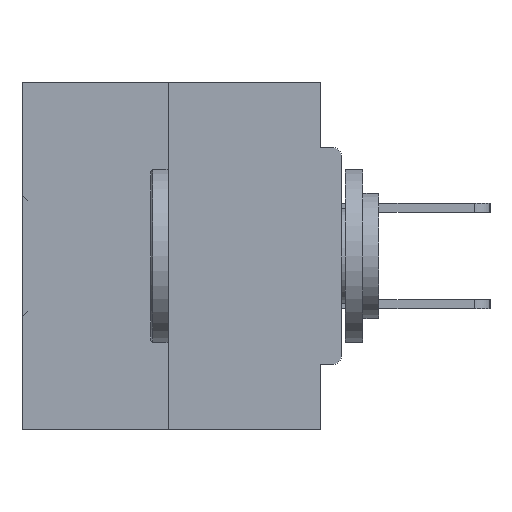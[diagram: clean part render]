
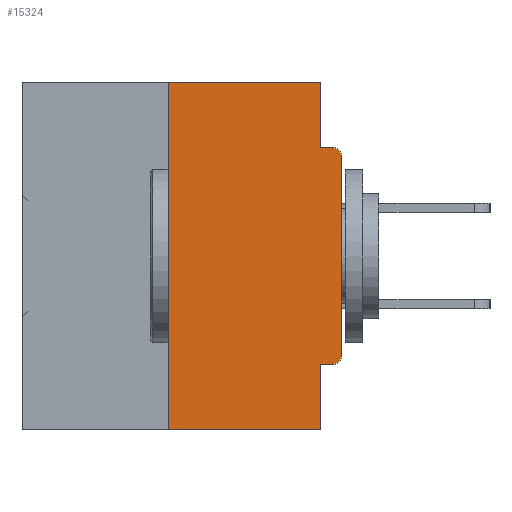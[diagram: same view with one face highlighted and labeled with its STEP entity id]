
A CAD part, left-side view. The second image highlights one B-rep face of the part: STEP entity #15324.
In plain terms, the highlighted planar face has unit normal (-1, 0, 0).
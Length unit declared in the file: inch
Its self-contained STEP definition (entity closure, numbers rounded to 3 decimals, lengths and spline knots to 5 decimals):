
#366 = LINE ( 'NONE', #34120, #34697 ) ;
#752 = AXIS2_PLACEMENT_3D ( 'NONE', #9094, #35102, #16743 ) ;
#790 = DIRECTION ( 'NONE',  ( 0., 1., 0. ) ) ;
#894 = DIRECTION ( 'NONE',  ( 0., -1., 0. ) ) ;
#1002 = ORIENTED_EDGE ( 'NONE', *, *, #1073, .F. ) ;
#1073 = EDGE_CURVE ( 'NONE', #8183, #37751, #38777, .T. ) ;
#2745 = EDGE_CURVE ( 'NONE', #17777, #28330, #366, .T. ) ;
#3215 = AXIS2_PLACEMENT_3D ( 'NONE', #20909, #6775, #28810 ) ;
#4293 = EDGE_CURVE ( 'NONE', #5166, #22107, #28750, .T. ) ;
#4902 = CARTESIAN_POINT ( 'NONE',  ( 0., 0.46, -0.5 ) ) ;
#5001 = DIRECTION ( 'NONE',  ( 0., 0., 1. ) ) ;
#5049 = AXIS2_PLACEMENT_3D ( 'NONE', #6238, #16967, #46202 ) ;
#5166 = VERTEX_POINT ( 'NONE', #45903 ) ;
#6108 = VECTOR ( 'NONE', #5001, 39.37008 ) ;
#6238 = CARTESIAN_POINT ( 'NONE',  ( 0., 0.46, 0. ) ) ;
#6361 = ORIENTED_EDGE ( 'NONE', *, *, #19238, .F. ) ;
#6560 = VERTEX_POINT ( 'NONE', #32976 ) ;
#6732 = CARTESIAN_POINT ( 'NONE',  ( 0., 0.031, -0.0935 ) ) ;
#6775 = DIRECTION ( 'NONE',  ( -1., 0., 0. ) ) ;
#7239 = EDGE_CURVE ( 'NONE', #24102, #6560, #45724, .T. ) ;
#7596 = EDGE_CURVE ( 'NONE', #8183, #22107, #18834, .T. ) ;
#7931 = VECTOR ( 'NONE', #894, 39.37008 ) ;
#8078 = LINE ( 'NONE', #15878, #11506 ) ;
#8183 = VERTEX_POINT ( 'NONE', #12443 ) ;
#8232 = CARTESIAN_POINT ( 'NONE',  ( 0., 0.031, 0. ) ) ;
#9094 = CARTESIAN_POINT ( 'NONE',  ( 0., 0.015, -0.3915 ) ) ;
#9449 = ORIENTED_EDGE ( 'NONE', *, *, #27895, .T. ) ;
#9565 = CARTESIAN_POINT ( 'NONE',  ( 0., 0.031, -0.5 ) ) ;
#11238 = ORIENTED_EDGE ( 'NONE', *, *, #7596, .T. ) ;
#11506 = VECTOR ( 'NONE', #44979, 39.37008 ) ;
#12329 = CARTESIAN_POINT ( 'NONE',  ( 0., 0.25, 0. ) ) ;
#12443 = CARTESIAN_POINT ( 'NONE',  ( 0., 0.25, -0.5 ) ) ;
#13688 = DIRECTION ( 'NONE',  ( 0., 0., -1. ) ) ;
#14679 = VERTEX_POINT ( 'NONE', #15962 ) ;
#15324 = ADVANCED_FACE ( 'NONE', ( #37534 ), #31179, .F. ) ;
#15878 = CARTESIAN_POINT ( 'NONE',  ( 0., 0.031, 0. ) ) ;
#15962 = CARTESIAN_POINT ( 'NONE',  ( 0., 0.015, -0.4065 ) ) ;
#16018 = CARTESIAN_POINT ( 'NONE',  ( 0., 0.46, 0. ) ) ;
#16743 = DIRECTION ( 'NONE',  ( 0., 0., -1. ) ) ;
#16967 = DIRECTION ( 'NONE',  ( 1., 0., 0. ) ) ;
#17101 = CARTESIAN_POINT ( 'NONE',  ( 0., 0., 0. ) ) ;
#17777 = VERTEX_POINT ( 'NONE', #6732 ) ;
#18155 = ORIENTED_EDGE ( 'NONE', *, *, #26161, .F. ) ;
#18808 = EDGE_LOOP ( 'NONE', ( #18155, #1002, #11238, #30719, #33522, #9449, #39337, #42216, #21099, #6361 ) ) ;
#18834 = LINE ( 'NONE', #4902, #7931 ) ;
#19238 = EDGE_CURVE ( 'NONE', #31193, #17777, #8078, .T. ) ;
#19810 = DIRECTION ( 'NONE',  ( 0., -1., 0. ) ) ;
#20909 = CARTESIAN_POINT ( 'NONE',  ( 0., 0.015, -0.1085 ) ) ;
#21099 = ORIENTED_EDGE ( 'NONE', *, *, #2745, .F. ) ;
#21401 = CARTESIAN_POINT ( 'NONE',  ( 0., 0., -0.3915 ) ) ;
#22107 = VERTEX_POINT ( 'NONE', #40289 ) ;
#22546 = VECTOR ( 'NONE', #13688, 39.37008 ) ;
#22756 = CARTESIAN_POINT ( 'NONE',  ( 0., 0., -0.4065 ) ) ;
#23541 = LINE ( 'NONE', #16018, #34956 ) ;
#24102 = VERTEX_POINT ( 'NONE', #21401 ) ;
#24455 = CARTESIAN_POINT ( 'NONE',  ( 0., 0.25, 0. ) ) ;
#26161 = EDGE_CURVE ( 'NONE', #37751, #31193, #23541, .T. ) ;
#27895 = EDGE_CURVE ( 'NONE', #14679, #24102, #35081, .T. ) ;
#28124 = LINE ( 'NONE', #22756, #32124 ) ;
#28330 = VERTEX_POINT ( 'NONE', #41328 ) ;
#28750 = LINE ( 'NONE', #9565, #22546 ) ;
#28810 = DIRECTION ( 'NONE',  ( 0., 0., -1. ) ) ;
#30719 = ORIENTED_EDGE ( 'NONE', *, *, #4293, .F. ) ;
#31179 = PLANE ( 'NONE',  #5049 ) ;
#31193 = VERTEX_POINT ( 'NONE', #8232 ) ;
#31375 = VECTOR ( 'NONE', #46331, 39.37008 ) ;
#32124 = VECTOR ( 'NONE', #790, 39.37008 ) ;
#32976 = CARTESIAN_POINT ( 'NONE',  ( 0., 0., -0.1085 ) ) ;
#33522 = ORIENTED_EDGE ( 'NONE', *, *, #45069, .F. ) ;
#34120 = CARTESIAN_POINT ( 'NONE',  ( 0., 0., -0.0935 ) ) ;
#34697 = VECTOR ( 'NONE', #19810, 39.37008 ) ;
#34721 = DIRECTION ( 'NONE',  ( 0., -1., 0. ) ) ;
#34956 = VECTOR ( 'NONE', #34721, 39.37008 ) ;
#35081 = CIRCLE ( 'NONE', #752, 0.015 ) ;
#35102 = DIRECTION ( 'NONE',  ( -1., 0., 0. ) ) ;
#37534 = FACE_OUTER_BOUND ( 'NONE', #18808, .T. ) ;
#37751 = VERTEX_POINT ( 'NONE', #24455 ) ;
#38777 = LINE ( 'NONE', #12329, #6108 ) ;
#39337 = ORIENTED_EDGE ( 'NONE', *, *, #7239, .T. ) ;
#40289 = CARTESIAN_POINT ( 'NONE',  ( 0., 0.031, -0.5 ) ) ;
#41328 = CARTESIAN_POINT ( 'NONE',  ( 0., 0.015, -0.0935 ) ) ;
#41790 = EDGE_CURVE ( 'NONE', #6560, #28330, #43940, .T. ) ;
#42216 = ORIENTED_EDGE ( 'NONE', *, *, #41790, .T. ) ;
#43940 = CIRCLE ( 'NONE', #3215, 0.015 ) ;
#44979 = DIRECTION ( 'NONE',  ( 0., 0., -1. ) ) ;
#45069 = EDGE_CURVE ( 'NONE', #14679, #5166, #28124, .T. ) ;
#45724 = LINE ( 'NONE', #17101, #31375 ) ;
#45903 = CARTESIAN_POINT ( 'NONE',  ( 0., 0.031, -0.4065 ) ) ;
#46202 = DIRECTION ( 'NONE',  ( 0., 0., -1. ) ) ;
#46331 = DIRECTION ( 'NONE',  ( 0., 0., 1. ) ) ;
